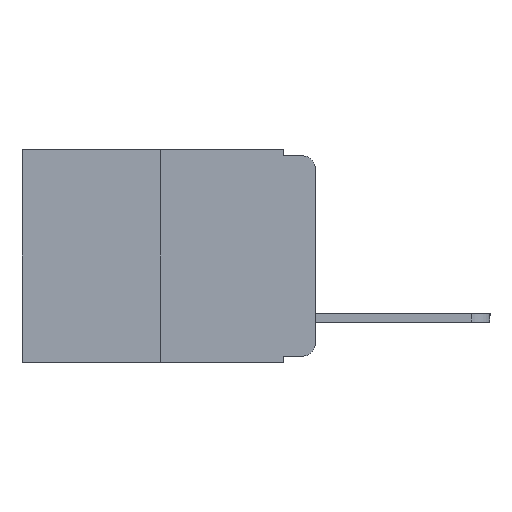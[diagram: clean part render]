
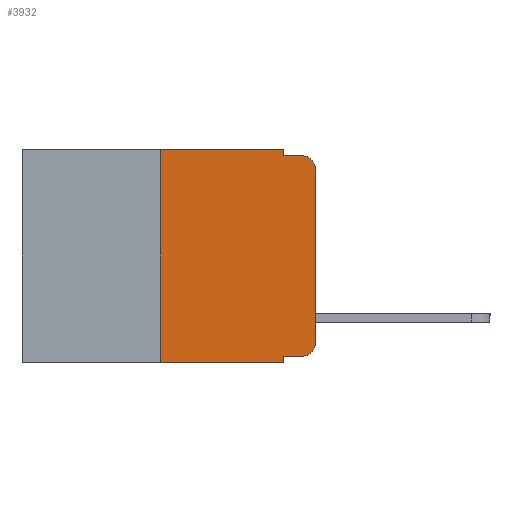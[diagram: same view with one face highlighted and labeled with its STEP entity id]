
A CAD part, left-side view. The second image highlights one B-rep face of the part: STEP entity #3932.
In plain terms, the highlighted planar face has unit normal (-1, 0, 0).
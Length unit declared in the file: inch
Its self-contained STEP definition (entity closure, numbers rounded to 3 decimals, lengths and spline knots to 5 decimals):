
#24 = VERTEX_POINT ( 'NONE', #14751 ) ;
#31 = CARTESIAN_POINT ( 'NONE',  ( 0., 0.051, -0.01 ) ) ;
#40 = ORIENTED_EDGE ( 'NONE', *, *, #21312, .F. ) ;
#68 = VERTEX_POINT ( 'NONE', #3581 ) ;
#268 = ORIENTED_EDGE ( 'NONE', *, *, #18950, .T. ) ;
#493 = CARTESIAN_POINT ( 'NONE',  ( 0., 0.051, -0.343 ) ) ;
#903 = CARTESIAN_POINT ( 'NONE',  ( 0., 0.02, -0.03 ) ) ;
#1275 = ORIENTED_EDGE ( 'NONE', *, *, #9495, .F. ) ;
#1316 = ORIENTED_EDGE ( 'NONE', *, *, #2641, .T. ) ;
#1457 = VECTOR ( 'NONE', #24071, 39.37008 ) ;
#1508 = LINE ( 'NONE', #11424, #16599 ) ;
#1616 = LINE ( 'NONE', #1955, #15539 ) ;
#1920 = DIRECTION ( 'NONE',  ( 0., 0., 1. ) ) ;
#1955 = CARTESIAN_POINT ( 'NONE',  ( 0., 0.473, -0.343 ) ) ;
#1970 = VERTEX_POINT ( 'NONE', #5618 ) ;
#2101 = ORIENTED_EDGE ( 'NONE', *, *, #16580, .T. ) ;
#2641 = EDGE_CURVE ( 'NONE', #5897, #24, #1508, .T. ) ;
#3426 = DIRECTION ( 'NONE',  ( 0., 0., -1. ) ) ;
#3581 = CARTESIAN_POINT ( 'NONE',  ( 0., 0.02, -0.01 ) ) ;
#3591 = EDGE_CURVE ( 'NONE', #20246, #19566, #14824, .T. ) ;
#3910 = VERTEX_POINT ( 'NONE', #15942 ) ;
#3932 = ADVANCED_FACE ( 'NONE', ( #10374 ), #3985, .F. ) ;
#3985 = PLANE ( 'NONE',  #16720 ) ;
#4437 = DIRECTION ( 'NONE',  ( 1., 0., 0. ) ) ;
#4464 = CARTESIAN_POINT ( 'NONE',  ( 0., 0.473, 0. ) ) ;
#4735 = VECTOR ( 'NONE', #21285, 39.37008 ) ;
#4860 = DIRECTION ( 'NONE',  ( -1., 0., 0. ) ) ;
#5130 = CARTESIAN_POINT ( 'NONE',  ( 0., 0.02, -0.313 ) ) ;
#5342 = EDGE_CURVE ( 'NONE', #14656, #68, #8810, .T. ) ;
#5618 = CARTESIAN_POINT ( 'NONE',  ( 0., 0., -0.313 ) ) ;
#5770 = DIRECTION ( 'NONE',  ( 0., -1., 0. ) ) ;
#5897 = VERTEX_POINT ( 'NONE', #13207 ) ;
#6165 = LINE ( 'NONE', #24324, #16226 ) ;
#7070 = DIRECTION ( 'NONE',  ( 0., 0., -1. ) ) ;
#7471 = DIRECTION ( 'NONE',  ( 0., -1., 0. ) ) ;
#7691 = EDGE_LOOP ( 'NONE', ( #18806, #23128, #18122, #23000, #20605, #40, #268, #1275, #1316, #2101 ) ) ;
#7894 = AXIS2_PLACEMENT_3D ( 'NONE', #5130, #18337, #7070 ) ;
#8180 = CARTESIAN_POINT ( 'NONE',  ( 0., 0., 0. ) ) ;
#8415 = AXIS2_PLACEMENT_3D ( 'NONE', #903, #4860, #9822 ) ;
#8810 = CIRCLE ( 'NONE', #8415, 0.02 ) ;
#8820 = EDGE_CURVE ( 'NONE', #3910, #20246, #15968, .T. ) ;
#9136 = VERTEX_POINT ( 'NONE', #493 ) ;
#9495 = EDGE_CURVE ( 'NONE', #5897, #9136, #6165, .T. ) ;
#9822 = DIRECTION ( 'NONE',  ( 0., 0., -1. ) ) ;
#10374 = FACE_OUTER_BOUND ( 'NONE', #7691, .T. ) ;
#10997 = LINE ( 'NONE', #22489, #22975 ) ;
#11009 = DIRECTION ( 'NONE',  ( 0., -1., 0. ) ) ;
#11424 = CARTESIAN_POINT ( 'NONE',  ( 0., 0.051, -0.333 ) ) ;
#11928 = DIRECTION ( 'NONE',  ( 0., 0., 1. ) ) ;
#13159 = DIRECTION ( 'NONE',  ( 0., 0., -1. ) ) ;
#13207 = CARTESIAN_POINT ( 'NONE',  ( 0., 0.051, -0.333 ) ) ;
#14656 = VERTEX_POINT ( 'NONE', #18580 ) ;
#14751 = CARTESIAN_POINT ( 'NONE',  ( 0., 0.02, -0.333 ) ) ;
#14824 = LINE ( 'NONE', #21613, #4735 ) ;
#15539 = VECTOR ( 'NONE', #5770, 39.37008 ) ;
#15942 = CARTESIAN_POINT ( 'NONE',  ( 0., 0.25, 0. ) ) ;
#15968 = LINE ( 'NONE', #22198, #1457 ) ;
#16226 = VECTOR ( 'NONE', #13159, 39.37008 ) ;
#16288 = VECTOR ( 'NONE', #1920, 39.37008 ) ;
#16580 = EDGE_CURVE ( 'NONE', #24, #1970, #22115, .T. ) ;
#16599 = VECTOR ( 'NONE', #11009, 39.37008 ) ;
#16720 = AXIS2_PLACEMENT_3D ( 'NONE', #4464, #4437, #3426 ) ;
#16731 = EDGE_CURVE ( 'NONE', #19566, #68, #10997, .T. ) ;
#18122 = ORIENTED_EDGE ( 'NONE', *, *, #16731, .F. ) ;
#18330 = VECTOR ( 'NONE', #11928, 39.37008 ) ;
#18337 = DIRECTION ( 'NONE',  ( -1., 0., 0. ) ) ;
#18580 = CARTESIAN_POINT ( 'NONE',  ( 0., 0., -0.03 ) ) ;
#18806 = ORIENTED_EDGE ( 'NONE', *, *, #21451, .T. ) ;
#18950 = EDGE_CURVE ( 'NONE', #23530, #9136, #1616, .T. ) ;
#19009 = CARTESIAN_POINT ( 'NONE',  ( 0., 0.051, 0. ) ) ;
#19566 = VERTEX_POINT ( 'NONE', #31 ) ;
#20246 = VERTEX_POINT ( 'NONE', #19009 ) ;
#20593 = CARTESIAN_POINT ( 'NONE',  ( 0., 0.25, -0.343 ) ) ;
#20605 = ORIENTED_EDGE ( 'NONE', *, *, #8820, .F. ) ;
#21285 = DIRECTION ( 'NONE',  ( 0., 0., -1. ) ) ;
#21312 = EDGE_CURVE ( 'NONE', #23530, #3910, #21871, .T. ) ;
#21451 = EDGE_CURVE ( 'NONE', #1970, #14656, #22716, .T. ) ;
#21613 = CARTESIAN_POINT ( 'NONE',  ( 0., 0.051, 0. ) ) ;
#21871 = LINE ( 'NONE', #22619, #16288 ) ;
#22115 = CIRCLE ( 'NONE', #7894, 0.02 ) ;
#22198 = CARTESIAN_POINT ( 'NONE',  ( 0., 0.473, 0. ) ) ;
#22489 = CARTESIAN_POINT ( 'NONE',  ( 0., 0.051, -0.01 ) ) ;
#22619 = CARTESIAN_POINT ( 'NONE',  ( 0., 0.25, 0. ) ) ;
#22716 = LINE ( 'NONE', #8180, #18330 ) ;
#22975 = VECTOR ( 'NONE', #7471, 39.37008 ) ;
#23000 = ORIENTED_EDGE ( 'NONE', *, *, #3591, .F. ) ;
#23128 = ORIENTED_EDGE ( 'NONE', *, *, #5342, .T. ) ;
#23530 = VERTEX_POINT ( 'NONE', #20593 ) ;
#24071 = DIRECTION ( 'NONE',  ( 0., -1., 0. ) ) ;
#24324 = CARTESIAN_POINT ( 'NONE',  ( 0., 0.051, 0. ) ) ;
